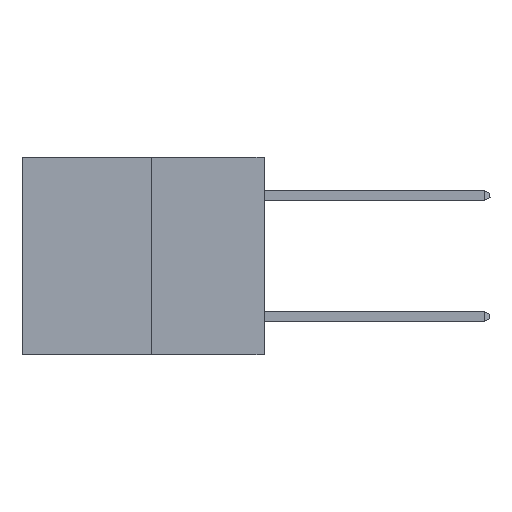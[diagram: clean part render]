
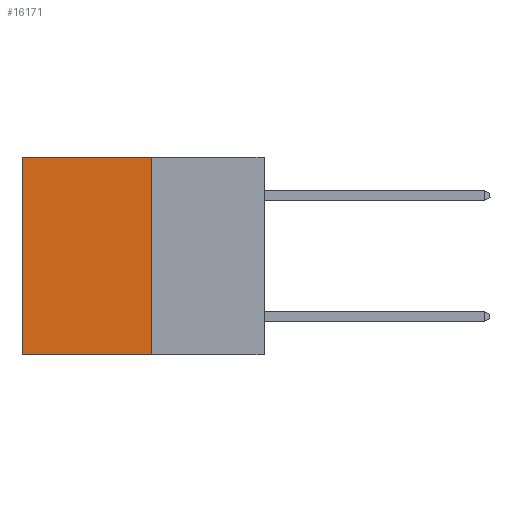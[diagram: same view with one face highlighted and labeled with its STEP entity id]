
A CAD part, left-side view. The second image highlights one B-rep face of the part: STEP entity #16171.
In plain terms, the highlighted planar face has unit normal (-1, 0, 0).
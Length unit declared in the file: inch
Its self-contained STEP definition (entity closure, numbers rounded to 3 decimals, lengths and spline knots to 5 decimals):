
#1784 = CARTESIAN_POINT ( 'NONE',  ( 0.3165, 0.28, 0. ) ) ;
#2126 = AXIS2_PLACEMENT_3D ( 'NONE', #15572, #21459, #23363 ) ;
#3703 = DIRECTION ( 'NONE',  ( 0., 1., 0. ) ) ;
#5244 = PLANE ( 'NONE',  #2126 ) ;
#6258 = CARTESIAN_POINT ( 'NONE',  ( 0.3165, 0.28, -0.49 ) ) ;
#6421 = LINE ( 'NONE', #15595, #18770 ) ;
#6879 = EDGE_CURVE ( 'NONE', #16162, #7089, #25220, .T. ) ;
#7089 = VERTEX_POINT ( 'NONE', #6258 ) ;
#8813 = CARTESIAN_POINT ( 'NONE',  ( 0.3165, 0.6, 0. ) ) ;
#9133 = VECTOR ( 'NONE', #16539, 39.37008 ) ;
#10863 = EDGE_CURVE ( 'NONE', #24478, #14709, #16286, .T. ) ;
#11417 = CARTESIAN_POINT ( 'NONE',  ( 0.3165, 0.6, -0.49 ) ) ;
#13416 = DIRECTION ( 'NONE',  ( 0., 0., -1. ) ) ;
#13802 = VECTOR ( 'NONE', #13416, 39.37008 ) ;
#14697 = CARTESIAN_POINT ( 'NONE',  ( 0.3165, 0.28, -0.49 ) ) ;
#14709 = VERTEX_POINT ( 'NONE', #16394 ) ;
#14710 = DIRECTION ( 'NONE',  ( 0., 1., 0. ) ) ;
#14974 = EDGE_LOOP ( 'NONE', ( #19623, #21527, #19781, #24520 ) ) ;
#15410 = FACE_OUTER_BOUND ( 'NONE', #14974, .T. ) ;
#15572 = CARTESIAN_POINT ( 'NONE',  ( 0.3165, 0.28, -0.49 ) ) ;
#15595 = CARTESIAN_POINT ( 'NONE',  ( 0.3165, 0.28, -0.49 ) ) ;
#16162 = VERTEX_POINT ( 'NONE', #1784 ) ;
#16171 = ADVANCED_FACE ( 'NONE', ( #15410 ), #5244, .F. ) ;
#16286 = LINE ( 'NONE', #11417, #13802 ) ;
#16394 = CARTESIAN_POINT ( 'NONE',  ( 0.3165, 0.6, -0.49 ) ) ;
#16539 = DIRECTION ( 'NONE',  ( 0., 0., -1. ) ) ;
#17249 = VECTOR ( 'NONE', #14710, 39.37008 ) ;
#17554 = LINE ( 'NONE', #24462, #17249 ) ;
#18770 = VECTOR ( 'NONE', #3703, 39.37008 ) ;
#19623 = ORIENTED_EDGE ( 'NONE', *, *, #10863, .T. ) ;
#19781 = ORIENTED_EDGE ( 'NONE', *, *, #6879, .F. ) ;
#21459 = DIRECTION ( 'NONE',  ( 1., 0., 0. ) ) ;
#21496 = EDGE_CURVE ( 'NONE', #7089, #14709, #6421, .T. ) ;
#21527 = ORIENTED_EDGE ( 'NONE', *, *, #21496, .F. ) ;
#21728 = EDGE_CURVE ( 'NONE', #16162, #24478, #17554, .T. ) ;
#23363 = DIRECTION ( 'NONE',  ( 0., 0., -1. ) ) ;
#24462 = CARTESIAN_POINT ( 'NONE',  ( 0.3165, 0.28, 0. ) ) ;
#24478 = VERTEX_POINT ( 'NONE', #8813 ) ;
#24520 = ORIENTED_EDGE ( 'NONE', *, *, #21728, .T. ) ;
#25220 = LINE ( 'NONE', #14697, #9133 ) ;
